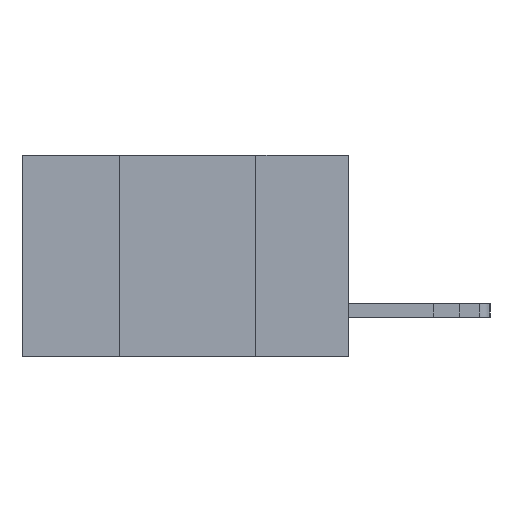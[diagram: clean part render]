
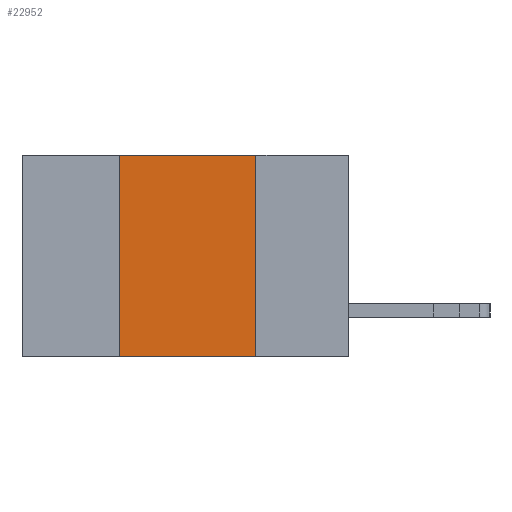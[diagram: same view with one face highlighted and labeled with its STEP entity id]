
A CAD part, left-side view. The second image highlights one B-rep face of the part: STEP entity #22952.
In plain terms, the highlighted planar face has unit normal (-1, 0, 0).
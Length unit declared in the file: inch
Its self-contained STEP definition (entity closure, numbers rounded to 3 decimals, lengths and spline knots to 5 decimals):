
#267 = ORIENTED_EDGE ( 'NONE', *, *, #2017, .F. ) ;
#1495 = CARTESIAN_POINT ( 'NONE',  ( 0., 0.17, 0. ) ) ;
#2017 = EDGE_CURVE ( 'NONE', #11068, #4156, #22709, .T. ) ;
#4110 = EDGE_LOOP ( 'NONE', ( #267, #17155, #10865, #8459 ) ) ;
#4156 = VERTEX_POINT ( 'NONE', #12356 ) ;
#5263 = CARTESIAN_POINT ( 'NONE',  ( 0., 0.42, 0. ) ) ;
#6020 = EDGE_CURVE ( 'NONE', #20338, #11068, #15360, .T. ) ;
#7314 = DIRECTION ( 'NONE',  ( 0., 0., 1. ) ) ;
#7664 = EDGE_CURVE ( 'NONE', #15503, #20338, #13466, .T. ) ;
#7939 = PLANE ( 'NONE',  #20015 ) ;
#7978 = VECTOR ( 'NONE', #7314, 39.37008 ) ;
#8025 = DIRECTION ( 'NONE',  ( 1., 0., 0. ) ) ;
#8082 = CARTESIAN_POINT ( 'NONE',  ( 0., 0.6, 0. ) ) ;
#8459 = ORIENTED_EDGE ( 'NONE', *, *, #9025, .T. ) ;
#9025 = EDGE_CURVE ( 'NONE', #15503, #4156, #15031, .T. ) ;
#9822 = DIRECTION ( 'NONE',  ( 0., 0., -1. ) ) ;
#10865 = ORIENTED_EDGE ( 'NONE', *, *, #7664, .F. ) ;
#11068 = VERTEX_POINT ( 'NONE', #22186 ) ;
#11629 = VECTOR ( 'NONE', #9822, 39.37008 ) ;
#12356 = CARTESIAN_POINT ( 'NONE',  ( 0., 0.17, -0.37 ) ) ;
#13466 = LINE ( 'NONE', #5263, #7978 ) ;
#15031 = LINE ( 'NONE', #15788, #20563 ) ;
#15360 = LINE ( 'NONE', #8082, #20249 ) ;
#15503 = VERTEX_POINT ( 'NONE', #20077 ) ;
#15788 = CARTESIAN_POINT ( 'NONE',  ( 0., 0.6, -0.37 ) ) ;
#17155 = ORIENTED_EDGE ( 'NONE', *, *, #6020, .F. ) ;
#17898 = DIRECTION ( 'NONE',  ( 0., -1., 0. ) ) ;
#20015 = AXIS2_PLACEMENT_3D ( 'NONE', #20477, #8025, #22552 ) ;
#20077 = CARTESIAN_POINT ( 'NONE',  ( 0., 0.42, -0.37 ) ) ;
#20249 = VECTOR ( 'NONE', #20525, 39.37008 ) ;
#20338 = VERTEX_POINT ( 'NONE', #26282 ) ;
#20477 = CARTESIAN_POINT ( 'NONE',  ( 0., 0.6, 0. ) ) ;
#20525 = DIRECTION ( 'NONE',  ( 0., -1., 0. ) ) ;
#20563 = VECTOR ( 'NONE', #17898, 39.37008 ) ;
#21689 = FACE_OUTER_BOUND ( 'NONE', #4110, .T. ) ;
#22186 = CARTESIAN_POINT ( 'NONE',  ( 0., 0.17, 0. ) ) ;
#22552 = DIRECTION ( 'NONE',  ( 0., 0., -1. ) ) ;
#22709 = LINE ( 'NONE', #1495, #11629 ) ;
#22952 = ADVANCED_FACE ( 'NONE', ( #21689 ), #7939, .F. ) ;
#26282 = CARTESIAN_POINT ( 'NONE',  ( 0., 0.42, 0. ) ) ;
